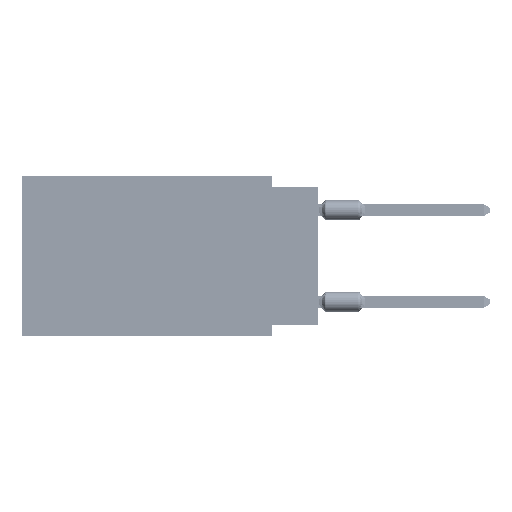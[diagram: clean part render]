
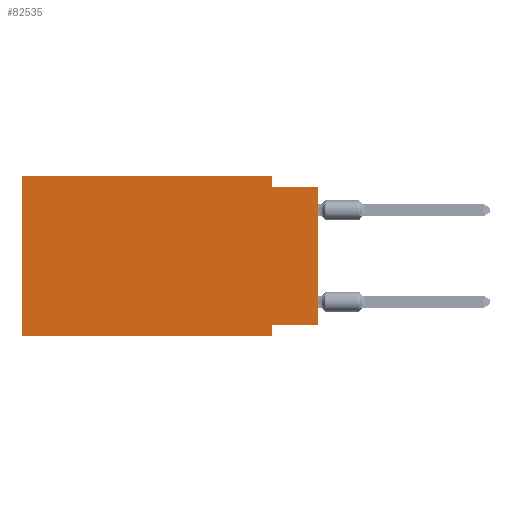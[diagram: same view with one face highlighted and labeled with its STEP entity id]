
A CAD part, left-side view. The second image highlights one B-rep face of the part: STEP entity #82535.
In plain terms, the highlighted planar face has unit normal (-1, 0, 0).
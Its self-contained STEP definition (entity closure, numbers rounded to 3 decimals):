
#373 = FACE_OUTER_BOUND ( 'NONE', #64199, .T. ) ;
#893 = VERTEX_POINT ( 'NONE', #92781 ) ;
#5541 = DIRECTION ( 'NONE',  ( 0., 1., 0. ) ) ;
#6280 = PLANE ( 'NONE',  #50683 ) ;
#7052 = DIRECTION ( 'NONE',  ( 0., 0., -1. ) ) ;
#7121 = VERTEX_POINT ( 'NONE', #66168 ) ;
#8067 = ORIENTED_EDGE ( 'NONE', *, *, #48508, .F. ) ;
#8211 = DIRECTION ( 'NONE',  ( 1., 0., 0. ) ) ;
#10025 = CARTESIAN_POINT ( 'NONE',  ( 0., 0., 0. ) ) ;
#12069 = ORIENTED_EDGE ( 'NONE', *, *, #72929, .T. ) ;
#13477 = VERTEX_POINT ( 'NONE', #43910 ) ;
#14896 = LINE ( 'NONE', #74315, #30075 ) ;
#14982 = LINE ( 'NONE', #10025, #15269 ) ;
#15269 = VECTOR ( 'NONE', #40448, 1000. ) ;
#16384 = EDGE_CURVE ( 'NONE', #66074, #61963, #96529, .T. ) ;
#17730 = VERTEX_POINT ( 'NONE', #32227 ) ;
#19576 = LINE ( 'NONE', #49512, #93899 ) ;
#20565 = ORIENTED_EDGE ( 'NONE', *, *, #77206, .F. ) ;
#21114 = VECTOR ( 'NONE', #64005, 1000. ) ;
#22600 = DIRECTION ( 'NONE',  ( 0., -1., 0. ) ) ;
#24792 = EDGE_CURVE ( 'NONE', #17730, #26291, #51158, .T. ) ;
#26291 = VERTEX_POINT ( 'NONE', #75239 ) ;
#29320 = CARTESIAN_POINT ( 'NONE',  ( 0., 0., -0.635 ) ) ;
#30075 = VECTOR ( 'NONE', #7052, 1000. ) ;
#30533 = VECTOR ( 'NONE', #89190, 1000. ) ;
#32227 = CARTESIAN_POINT ( 'NONE',  ( 0., 0., -8.255 ) ) ;
#32266 = VECTOR ( 'NONE', #45182, 1000. ) ;
#32934 = VERTEX_POINT ( 'NONE', #79253 ) ;
#34067 = LINE ( 'NONE', #72369, #21114 ) ;
#35279 = DIRECTION ( 'NONE',  ( 0., -1., 0. ) ) ;
#39737 = CARTESIAN_POINT ( 'NONE',  ( 0., 2.54, -8.89 ) ) ;
#40448 = DIRECTION ( 'NONE',  ( 0., 0., 1. ) ) ;
#41740 = ORIENTED_EDGE ( 'NONE', *, *, #63931, .T. ) ;
#43910 = CARTESIAN_POINT ( 'NONE',  ( 0., 16.383, -8.89 ) ) ;
#44586 = ORIENTED_EDGE ( 'NONE', *, *, #24792, .F. ) ;
#45182 = DIRECTION ( 'NONE',  ( 0., 0., -1. ) ) ;
#45433 = CARTESIAN_POINT ( 'NONE',  ( 0., 2.54, -0.635 ) ) ;
#47723 = ORIENTED_EDGE ( 'NONE', *, *, #69917, .F. ) ;
#48508 = EDGE_CURVE ( 'NONE', #893, #66074, #14896, .T. ) ;
#49512 = CARTESIAN_POINT ( 'NONE',  ( 0., 16.383, 0. ) ) ;
#50683 = AXIS2_PLACEMENT_3D ( 'NONE', #75481, #8211, #58785 ) ;
#51158 = LINE ( 'NONE', #65913, #65929 ) ;
#58785 = DIRECTION ( 'NONE',  ( 0., 0., -1. ) ) ;
#59399 = CARTESIAN_POINT ( 'NONE',  ( 0., 16.383, -8.89 ) ) ;
#61963 = VERTEX_POINT ( 'NONE', #63312 ) ;
#63312 = CARTESIAN_POINT ( 'NONE',  ( 0., 0., -0.635 ) ) ;
#63931 = EDGE_CURVE ( 'NONE', #13477, #32934, #89824, .T. ) ;
#64005 = DIRECTION ( 'NONE',  ( 0., 0., 1. ) ) ;
#64199 = EDGE_LOOP ( 'NONE', ( #12069, #75114, #8067, #20565, #47723, #41740, #73914, #44586 ) ) ;
#65913 = CARTESIAN_POINT ( 'NONE',  ( 0., 0., -8.255 ) ) ;
#65929 = VECTOR ( 'NONE', #5541, 1000. ) ;
#66074 = VERTEX_POINT ( 'NONE', #45433 ) ;
#66168 = CARTESIAN_POINT ( 'NONE',  ( 0., 16.383, 0. ) ) ;
#69917 = EDGE_CURVE ( 'NONE', #13477, #7121, #34067, .T. ) ;
#72369 = CARTESIAN_POINT ( 'NONE',  ( 0., 16.383, 0. ) ) ;
#72929 = EDGE_CURVE ( 'NONE', #17730, #61963, #14982, .T. ) ;
#73914 = ORIENTED_EDGE ( 'NONE', *, *, #84603, .F. ) ;
#74315 = CARTESIAN_POINT ( 'NONE',  ( 0., 2.54, 0. ) ) ;
#75114 = ORIENTED_EDGE ( 'NONE', *, *, #16384, .F. ) ;
#75239 = CARTESIAN_POINT ( 'NONE',  ( 0., 2.54, -8.255 ) ) ;
#75481 = CARTESIAN_POINT ( 'NONE',  ( 0., 16.383, 0. ) ) ;
#77206 = EDGE_CURVE ( 'NONE', #7121, #893, #19576, .T. ) ;
#79253 = CARTESIAN_POINT ( 'NONE',  ( 0., 2.54, -8.89 ) ) ;
#82535 = ADVANCED_FACE ( 'NONE', ( #373 ), #6280, .F. ) ;
#82787 = VECTOR ( 'NONE', #22600, 1000. ) ;
#84603 = EDGE_CURVE ( 'NONE', #26291, #32934, #84895, .T. ) ;
#84895 = LINE ( 'NONE', #39737, #32266 ) ;
#89190 = DIRECTION ( 'NONE',  ( 0., -1., 0. ) ) ;
#89824 = LINE ( 'NONE', #59399, #82787 ) ;
#92781 = CARTESIAN_POINT ( 'NONE',  ( 0., 2.54, 0. ) ) ;
#93899 = VECTOR ( 'NONE', #35279, 1000. ) ;
#96529 = LINE ( 'NONE', #29320, #30533 ) ;
